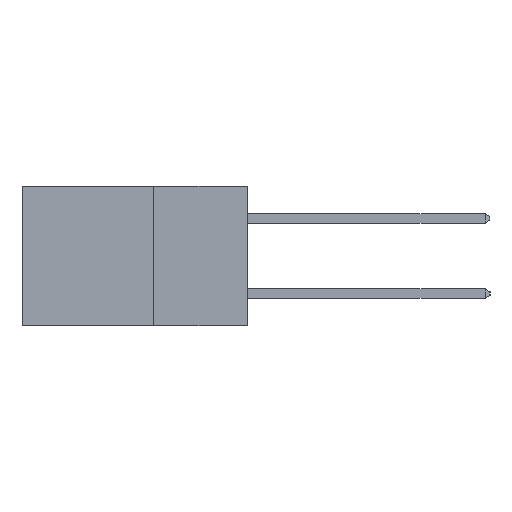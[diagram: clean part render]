
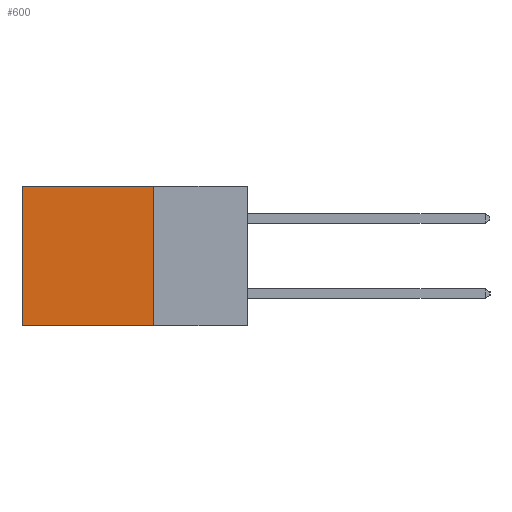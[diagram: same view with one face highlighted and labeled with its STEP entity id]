
A CAD part, left-side view. The second image highlights one B-rep face of the part: STEP entity #600.
In plain terms, the highlighted planar face has unit normal (-1, 0, 0).
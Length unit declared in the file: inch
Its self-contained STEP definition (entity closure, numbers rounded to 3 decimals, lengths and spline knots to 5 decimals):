
#70 = VECTOR ( 'NONE', #3005, 39.37008 ) ;
#202 = CARTESIAN_POINT ( 'NONE',  ( 0.2615, 0.25, -0.37 ) ) ;
#600 = ADVANCED_FACE ( 'NONE', ( #4925 ), #12475, .F. ) ;
#928 = VERTEX_POINT ( 'NONE', #3313 ) ;
#1054 = VERTEX_POINT ( 'NONE', #9352 ) ;
#1312 = CARTESIAN_POINT ( 'NONE',  ( 0.2615, 0.25, 0. ) ) ;
#2447 = ORIENTED_EDGE ( 'NONE', *, *, #6077, .T. ) ;
#3005 = DIRECTION ( 'NONE',  ( 0., 0., -1. ) ) ;
#3048 = CARTESIAN_POINT ( 'NONE',  ( 0.2615, 0.6, -0.37 ) ) ;
#3115 = CARTESIAN_POINT ( 'NONE',  ( 0.2615, 0.25, -0.37 ) ) ;
#3196 = ORIENTED_EDGE ( 'NONE', *, *, #3411, .F. ) ;
#3313 = CARTESIAN_POINT ( 'NONE',  ( 0.2615, 0.6, 0. ) ) ;
#3411 = EDGE_CURVE ( 'NONE', #10322, #11250, #4226, .T. ) ;
#3821 = LINE ( 'NONE', #3833, #9222 ) ;
#3833 = CARTESIAN_POINT ( 'NONE',  ( 0.2615, 0.25, 0. ) ) ;
#4226 = LINE ( 'NONE', #11010, #9950 ) ;
#4925 = FACE_OUTER_BOUND ( 'NONE', #13172, .T. ) ;
#6077 = EDGE_CURVE ( 'NONE', #10322, #928, #3821, .T. ) ;
#6941 = ORIENTED_EDGE ( 'NONE', *, *, #13637, .T. ) ;
#7419 = LINE ( 'NONE', #3115, #12295 ) ;
#8077 = EDGE_CURVE ( 'NONE', #11250, #1054, #7419, .T. ) ;
#8731 = DIRECTION ( 'NONE',  ( 0., 1., 0. ) ) ;
#9222 = VECTOR ( 'NONE', #8731, 39.37008 ) ;
#9352 = CARTESIAN_POINT ( 'NONE',  ( 0.2615, 0.6, -0.37 ) ) ;
#9411 = DIRECTION ( 'NONE',  ( 1., 0., 0. ) ) ;
#9645 = DIRECTION ( 'NONE',  ( 0., 0., -1. ) ) ;
#9950 = VECTOR ( 'NONE', #10984, 39.37008 ) ;
#10322 = VERTEX_POINT ( 'NONE', #1312 ) ;
#10339 = ORIENTED_EDGE ( 'NONE', *, *, #8077, .F. ) ;
#10621 = CARTESIAN_POINT ( 'NONE',  ( 0.2615, 0.25, -0.37 ) ) ;
#10984 = DIRECTION ( 'NONE',  ( 0., 0., -1. ) ) ;
#11010 = CARTESIAN_POINT ( 'NONE',  ( 0.2615, 0.25, -0.37 ) ) ;
#11250 = VERTEX_POINT ( 'NONE', #202 ) ;
#11853 = LINE ( 'NONE', #3048, #70 ) ;
#12274 = DIRECTION ( 'NONE',  ( 0., 1., 0. ) ) ;
#12295 = VECTOR ( 'NONE', #12274, 39.37008 ) ;
#12475 = PLANE ( 'NONE',  #12719 ) ;
#12719 = AXIS2_PLACEMENT_3D ( 'NONE', #10621, #9411, #9645 ) ;
#13172 = EDGE_LOOP ( 'NONE', ( #6941, #10339, #3196, #2447 ) ) ;
#13637 = EDGE_CURVE ( 'NONE', #928, #1054, #11853, .T. ) ;
